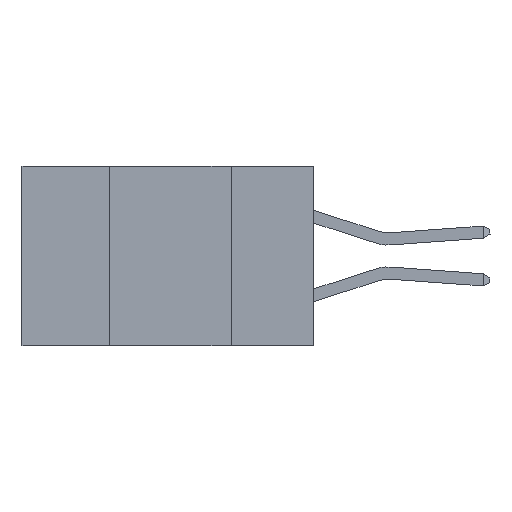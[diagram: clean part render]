
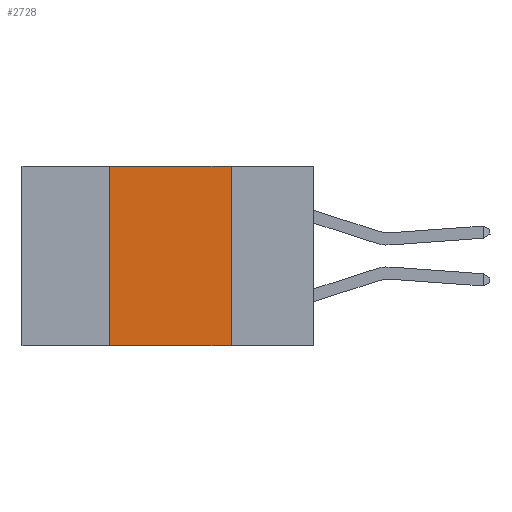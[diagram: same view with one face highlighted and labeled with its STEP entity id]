
A CAD part, left-side view. The second image highlights one B-rep face of the part: STEP entity #2728.
In plain terms, the highlighted planar face has unit normal (-1, 0, 0).
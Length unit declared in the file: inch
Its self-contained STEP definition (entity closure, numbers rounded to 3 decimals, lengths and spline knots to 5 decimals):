
#971 = PLANE ( 'NONE',  #8630 ) ;
#1628 = CARTESIAN_POINT ( 'NONE',  ( 0., 0.17, 0. ) ) ;
#1755 = VERTEX_POINT ( 'NONE', #4363 ) ;
#2111 = ORIENTED_EDGE ( 'NONE', *, *, #9743, .T. ) ;
#2616 = CARTESIAN_POINT ( 'NONE',  ( 0., 0.42, 0. ) ) ;
#2728 = ADVANCED_FACE ( 'NONE', ( #7258 ), #971, .F. ) ;
#3226 = CARTESIAN_POINT ( 'NONE',  ( 0., 0.17, 0. ) ) ;
#3750 = DIRECTION ( 'NONE',  ( 0., -1., 0. ) ) ;
#4070 = CARTESIAN_POINT ( 'NONE',  ( 0., 0.6, 0. ) ) ;
#4363 = CARTESIAN_POINT ( 'NONE',  ( 0., 0.42, -0.37 ) ) ;
#4900 = ORIENTED_EDGE ( 'NONE', *, *, #9516, .F. ) ;
#5060 = ORIENTED_EDGE ( 'NONE', *, *, #12932, .F. ) ;
#5540 = DIRECTION ( 'NONE',  ( 0., 0., -1. ) ) ;
#6118 = VECTOR ( 'NONE', #8626, 39.37008 ) ;
#6228 = CARTESIAN_POINT ( 'NONE',  ( 0., 0.17, -0.37 ) ) ;
#7258 = FACE_OUTER_BOUND ( 'NONE', #13846, .T. ) ;
#7439 = DIRECTION ( 'NONE',  ( 0., 0., -1. ) ) ;
#7706 = EDGE_CURVE ( 'NONE', #11567, #13573, #10576, .T. ) ;
#7740 = LINE ( 'NONE', #12838, #8202 ) ;
#8143 = DIRECTION ( 'NONE',  ( 0., -1., 0. ) ) ;
#8202 = VECTOR ( 'NONE', #3750, 39.37008 ) ;
#8626 = DIRECTION ( 'NONE',  ( 0., 0., 1. ) ) ;
#8630 = AXIS2_PLACEMENT_3D ( 'NONE', #8798, #15089, #7439 ) ;
#8798 = CARTESIAN_POINT ( 'NONE',  ( 0., 0.6, 0. ) ) ;
#9516 = EDGE_CURVE ( 'NONE', #13573, #14636, #14546, .T. ) ;
#9743 = EDGE_CURVE ( 'NONE', #1755, #14636, #7740, .T. ) ;
#10576 = LINE ( 'NONE', #4070, #11177 ) ;
#11177 = VECTOR ( 'NONE', #8143, 39.37008 ) ;
#11567 = VERTEX_POINT ( 'NONE', #2616 ) ;
#12838 = CARTESIAN_POINT ( 'NONE',  ( 0., 0.6, -0.37 ) ) ;
#12932 = EDGE_CURVE ( 'NONE', #1755, #11567, #15183, .T. ) ;
#13573 = VERTEX_POINT ( 'NONE', #3226 ) ;
#13846 = EDGE_LOOP ( 'NONE', ( #4900, #14614, #5060, #2111 ) ) ;
#14546 = LINE ( 'NONE', #1628, #14619 ) ;
#14614 = ORIENTED_EDGE ( 'NONE', *, *, #7706, .F. ) ;
#14619 = VECTOR ( 'NONE', #5540, 39.37008 ) ;
#14636 = VERTEX_POINT ( 'NONE', #6228 ) ;
#15089 = DIRECTION ( 'NONE',  ( 1., 0., 0. ) ) ;
#15183 = LINE ( 'NONE', #16531, #6118 ) ;
#16531 = CARTESIAN_POINT ( 'NONE',  ( 0., 0.42, 0. ) ) ;
